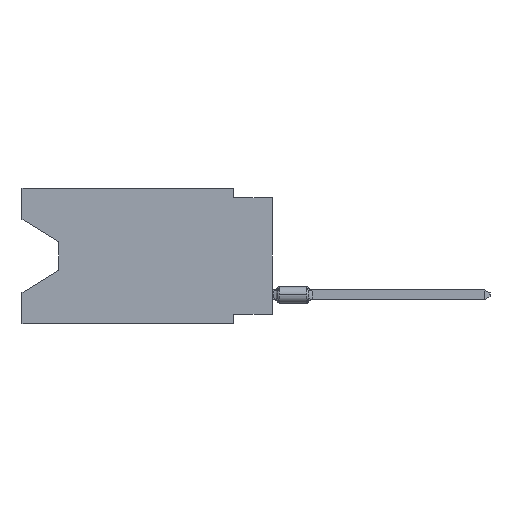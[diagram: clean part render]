
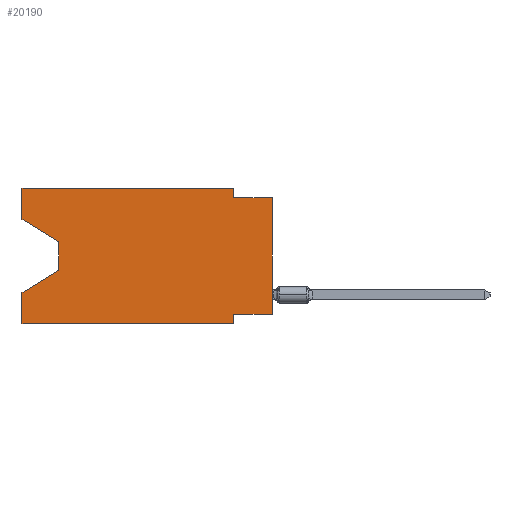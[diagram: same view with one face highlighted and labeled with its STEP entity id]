
A CAD part, left-side view. The second image highlights one B-rep face of the part: STEP entity #20190.
In plain terms, the highlighted planar face has unit normal (-1, 0, 0).
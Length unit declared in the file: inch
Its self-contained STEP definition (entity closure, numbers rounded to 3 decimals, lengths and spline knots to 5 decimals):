
#122 = DIRECTION ( 'NONE',  ( 1., 0., 0. ) ) ;
#225 = VERTEX_POINT ( 'NONE', #27370 ) ;
#745 = DIRECTION ( 'NONE',  ( 0., -1., 0. ) ) ;
#774 = EDGE_CURVE ( 'NONE', #6494, #20549, #3487, .T. ) ;
#804 = CARTESIAN_POINT ( 'NONE',  ( 0., 0.55, -0.212 ) ) ;
#823 = LINE ( 'NONE', #11103, #14821 ) ;
#1295 = CARTESIAN_POINT ( 'NONE',  ( 0., 0.1, 0. ) ) ;
#1515 = VERTEX_POINT ( 'NONE', #23912 ) ;
#1529 = VECTOR ( 'NONE', #745, 39.37008 ) ;
#1831 = ORIENTED_EDGE ( 'NONE', *, *, #3914, .T. ) ;
#1911 = LINE ( 'NONE', #8025, #27336 ) ;
#2476 = DIRECTION ( 'NONE',  ( 0., 0.855, -0.519 ) ) ;
#3200 = CARTESIAN_POINT ( 'NONE',  ( 0., 0.55, -0.138 ) ) ;
#3487 = LINE ( 'NONE', #24549, #3594 ) ;
#3594 = VECTOR ( 'NONE', #5571, 39.37008 ) ;
#3903 = CARTESIAN_POINT ( 'NONE',  ( 0., 0.645, -0.08025 ) ) ;
#3914 = EDGE_CURVE ( 'NONE', #19052, #15946, #823, .T. ) ;
#4032 = DIRECTION ( 'NONE',  ( 0., 0., -1. ) ) ;
#4033 = ORIENTED_EDGE ( 'NONE', *, *, #18845, .F. ) ;
#4048 = ORIENTED_EDGE ( 'NONE', *, *, #25530, .F. ) ;
#4270 = CARTESIAN_POINT ( 'NONE',  ( 0., 0.645, -0.35 ) ) ;
#4563 = LINE ( 'NONE', #804, #11563 ) ;
#4608 = LINE ( 'NONE', #8629, #23210 ) ;
#5013 = LINE ( 'NONE', #11118, #7530 ) ;
#5571 = DIRECTION ( 'NONE',  ( 0., 0., 1. ) ) ;
#6049 = ORIENTED_EDGE ( 'NONE', *, *, #10538, .F. ) ;
#6200 = ORIENTED_EDGE ( 'NONE', *, *, #22842, .F. ) ;
#6331 = VERTEX_POINT ( 'NONE', #16349 ) ;
#6494 = VERTEX_POINT ( 'NONE', #4270 ) ;
#7530 = VECTOR ( 'NONE', #13476, 39.37008 ) ;
#8025 = CARTESIAN_POINT ( 'NONE',  ( 0., 0., -0.325 ) ) ;
#8629 = CARTESIAN_POINT ( 'NONE',  ( 0., 0.645, -0.08025 ) ) ;
#9080 = CARTESIAN_POINT ( 'NONE',  ( 0., 0.645, -0.35 ) ) ;
#10082 = ORIENTED_EDGE ( 'NONE', *, *, #15200, .T. ) ;
#10185 = VECTOR ( 'NONE', #17441, 39.37008 ) ;
#10538 = EDGE_CURVE ( 'NONE', #23523, #225, #19796, .T. ) ;
#11103 = CARTESIAN_POINT ( 'NONE',  ( 0., 0., 0. ) ) ;
#11118 = CARTESIAN_POINT ( 'NONE',  ( 0., 0.1, 0. ) ) ;
#11199 = VECTOR ( 'NONE', #13650, 39.37008 ) ;
#11267 = DIRECTION ( 'NONE',  ( 0., -0.855, -0.519 ) ) ;
#11334 = EDGE_CURVE ( 'NONE', #18533, #1515, #5013, .T. ) ;
#11521 = AXIS2_PLACEMENT_3D ( 'NONE', #19000, #122, #4032 ) ;
#11563 = VECTOR ( 'NONE', #2476, 39.37008 ) ;
#11663 = EDGE_CURVE ( 'NONE', #12736, #20549, #4563, .T. ) ;
#11673 = LINE ( 'NONE', #3200, #12055 ) ;
#12055 = VECTOR ( 'NONE', #18027, 39.37008 ) ;
#12736 = VERTEX_POINT ( 'NONE', #26485 ) ;
#13238 = LINE ( 'NONE', #23749, #11199 ) ;
#13476 = DIRECTION ( 'NONE',  ( 0., 0., -1. ) ) ;
#13650 = DIRECTION ( 'NONE',  ( 0., -1., 0. ) ) ;
#13775 = VERTEX_POINT ( 'NONE', #14051 ) ;
#13836 = VERTEX_POINT ( 'NONE', #21329 ) ;
#14021 = DIRECTION ( 'NONE',  ( 0., 0., -1. ) ) ;
#14051 = CARTESIAN_POINT ( 'NONE',  ( 0., 0.55, -0.138 ) ) ;
#14559 = ORIENTED_EDGE ( 'NONE', *, *, #11334, .F. ) ;
#14821 = VECTOR ( 'NONE', #26052, 39.37008 ) ;
#15200 = EDGE_CURVE ( 'NONE', #23523, #13775, #4608, .T. ) ;
#15946 = VERTEX_POINT ( 'NONE', #21951 ) ;
#16190 = EDGE_LOOP ( 'NONE', ( #10082, #25752, #25886, #17851, #24158, #4033, #6200, #1831, #4048, #14559, #21553, #6049 ) ) ;
#16349 = CARTESIAN_POINT ( 'NONE',  ( 0., 0.1, -0.35 ) ) ;
#16484 = DIRECTION ( 'NONE',  ( 0., 1., 0. ) ) ;
#17386 = LINE ( 'NONE', #21809, #24458 ) ;
#17441 = DIRECTION ( 'NONE',  ( 0., 0., 1. ) ) ;
#17851 = ORIENTED_EDGE ( 'NONE', *, *, #774, .F. ) ;
#18027 = DIRECTION ( 'NONE',  ( 0., 0., -1. ) ) ;
#18533 = VERTEX_POINT ( 'NONE', #1295 ) ;
#18845 = EDGE_CURVE ( 'NONE', #13836, #6331, #20401, .T. ) ;
#19000 = CARTESIAN_POINT ( 'NONE',  ( 0., 0.645, 0. ) ) ;
#19052 = VERTEX_POINT ( 'NONE', #23008 ) ;
#19796 = LINE ( 'NONE', #23395, #10185 ) ;
#20190 = ADVANCED_FACE ( 'NONE', ( #21203 ), #27166, .F. ) ;
#20401 = LINE ( 'NONE', #22190, #22921 ) ;
#20549 = VERTEX_POINT ( 'NONE', #24503 ) ;
#21203 = FACE_OUTER_BOUND ( 'NONE', #16190, .T. ) ;
#21329 = CARTESIAN_POINT ( 'NONE',  ( 0., 0.1, -0.325 ) ) ;
#21553 = ORIENTED_EDGE ( 'NONE', *, *, #25488, .F. ) ;
#21809 = CARTESIAN_POINT ( 'NONE',  ( 0., 0., -0.025 ) ) ;
#21951 = CARTESIAN_POINT ( 'NONE',  ( 0., 0., -0.025 ) ) ;
#22092 = DIRECTION ( 'NONE',  ( 0., -1., 0. ) ) ;
#22190 = CARTESIAN_POINT ( 'NONE',  ( 0., 0.1, -0.35 ) ) ;
#22737 = LINE ( 'NONE', #9080, #1529 ) ;
#22842 = EDGE_CURVE ( 'NONE', #19052, #13836, #1911, .T. ) ;
#22921 = VECTOR ( 'NONE', #14021, 39.37008 ) ;
#23008 = CARTESIAN_POINT ( 'NONE',  ( 0., 0., -0.325 ) ) ;
#23210 = VECTOR ( 'NONE', #11267, 39.37008 ) ;
#23395 = CARTESIAN_POINT ( 'NONE',  ( 0., 0.645, 0. ) ) ;
#23523 = VERTEX_POINT ( 'NONE', #3903 ) ;
#23749 = CARTESIAN_POINT ( 'NONE',  ( 0., 0.645, 0. ) ) ;
#23912 = CARTESIAN_POINT ( 'NONE',  ( 0., 0.1, -0.025 ) ) ;
#24158 = ORIENTED_EDGE ( 'NONE', *, *, #27291, .T. ) ;
#24458 = VECTOR ( 'NONE', #22092, 39.37008 ) ;
#24503 = CARTESIAN_POINT ( 'NONE',  ( 0., 0.645, -0.26975 ) ) ;
#24549 = CARTESIAN_POINT ( 'NONE',  ( 0., 0.645, 0. ) ) ;
#24879 = EDGE_CURVE ( 'NONE', #13775, #12736, #11673, .T. ) ;
#25488 = EDGE_CURVE ( 'NONE', #225, #18533, #13238, .T. ) ;
#25530 = EDGE_CURVE ( 'NONE', #1515, #15946, #17386, .T. ) ;
#25752 = ORIENTED_EDGE ( 'NONE', *, *, #24879, .T. ) ;
#25886 = ORIENTED_EDGE ( 'NONE', *, *, #11663, .T. ) ;
#26052 = DIRECTION ( 'NONE',  ( 0., 0., 1. ) ) ;
#26485 = CARTESIAN_POINT ( 'NONE',  ( 0., 0.55, -0.212 ) ) ;
#27166 = PLANE ( 'NONE',  #11521 ) ;
#27291 = EDGE_CURVE ( 'NONE', #6494, #6331, #22737, .T. ) ;
#27336 = VECTOR ( 'NONE', #16484, 39.37008 ) ;
#27370 = CARTESIAN_POINT ( 'NONE',  ( 0., 0.645, 0. ) ) ;
